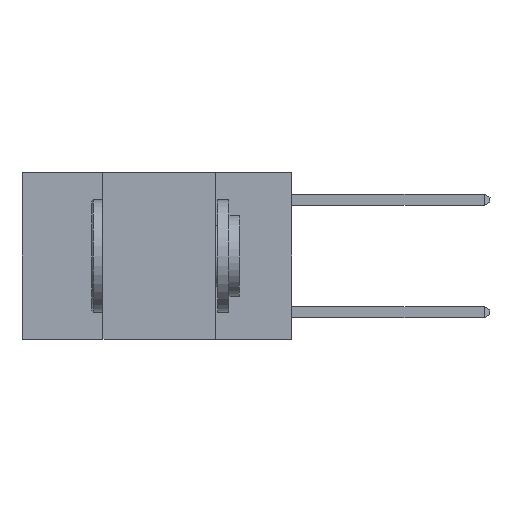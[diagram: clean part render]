
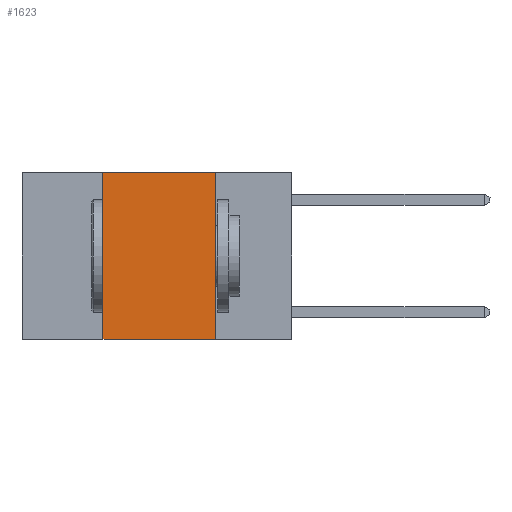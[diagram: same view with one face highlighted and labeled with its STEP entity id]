
A CAD part, left-side view. The second image highlights one B-rep face of the part: STEP entity #1623.
In plain terms, the highlighted planar face has unit normal (-1, 0, 0).
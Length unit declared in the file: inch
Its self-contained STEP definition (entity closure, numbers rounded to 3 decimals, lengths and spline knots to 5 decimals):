
#949 = CARTESIAN_POINT ( 'NONE',  ( 0., 0.17, 0. ) ) ;
#995 = CARTESIAN_POINT ( 'NONE',  ( 0., 0.6, -0.37 ) ) ;
#1240 = CARTESIAN_POINT ( 'NONE',  ( 0., 0.6, 0. ) ) ;
#1572 = DIRECTION ( 'NONE',  ( 0., 0., -1. ) ) ;
#1623 = ADVANCED_FACE ( 'NONE', ( #8697 ), #2121, .F. ) ;
#1650 = EDGE_CURVE ( 'NONE', #4309, #4981, #1725, .T. ) ;
#1725 = LINE ( 'NONE', #995, #6433 ) ;
#2109 = LINE ( 'NONE', #1240, #7111 ) ;
#2121 = PLANE ( 'NONE',  #3975 ) ;
#2131 = ORIENTED_EDGE ( 'NONE', *, *, #5411, .F. ) ;
#2407 = ORIENTED_EDGE ( 'NONE', *, *, #1650, .T. ) ;
#2868 = CARTESIAN_POINT ( 'NONE',  ( 0., 0.17, 0. ) ) ;
#3050 = VECTOR ( 'NONE', #1572, 39.37008 ) ;
#3256 = DIRECTION ( 'NONE',  ( 0., -1., 0. ) ) ;
#3333 = CARTESIAN_POINT ( 'NONE',  ( 0., 0.42, 0. ) ) ;
#3726 = ORIENTED_EDGE ( 'NONE', *, *, #3736, .F. ) ;
#3736 = EDGE_CURVE ( 'NONE', #5760, #6462, #2109, .T. ) ;
#3975 = AXIS2_PLACEMENT_3D ( 'NONE', #5078, #7504, #4783 ) ;
#4120 = CARTESIAN_POINT ( 'NONE',  ( 0., 0.17, -0.37 ) ) ;
#4208 = EDGE_LOOP ( 'NONE', ( #4667, #3726, #2131, #2407 ) ) ;
#4309 = VERTEX_POINT ( 'NONE', #5350 ) ;
#4667 = ORIENTED_EDGE ( 'NONE', *, *, #5664, .F. ) ;
#4783 = DIRECTION ( 'NONE',  ( 0., 0., -1. ) ) ;
#4833 = CARTESIAN_POINT ( 'NONE',  ( 0., 0.42, 0. ) ) ;
#4981 = VERTEX_POINT ( 'NONE', #4120 ) ;
#5078 = CARTESIAN_POINT ( 'NONE',  ( 0., 0.6, 0. ) ) ;
#5350 = CARTESIAN_POINT ( 'NONE',  ( 0., 0.42, -0.37 ) ) ;
#5354 = VECTOR ( 'NONE', #5598, 39.37008 ) ;
#5411 = EDGE_CURVE ( 'NONE', #4309, #5760, #9169, .T. ) ;
#5598 = DIRECTION ( 'NONE',  ( 0., 0., 1. ) ) ;
#5664 = EDGE_CURVE ( 'NONE', #6462, #4981, #8167, .T. ) ;
#5760 = VERTEX_POINT ( 'NONE', #3333 ) ;
#6433 = VECTOR ( 'NONE', #3256, 39.37008 ) ;
#6462 = VERTEX_POINT ( 'NONE', #2868 ) ;
#7111 = VECTOR ( 'NONE', #9450, 39.37008 ) ;
#7504 = DIRECTION ( 'NONE',  ( 1., 0., 0. ) ) ;
#8167 = LINE ( 'NONE', #949, #3050 ) ;
#8697 = FACE_OUTER_BOUND ( 'NONE', #4208, .T. ) ;
#9169 = LINE ( 'NONE', #4833, #5354 ) ;
#9450 = DIRECTION ( 'NONE',  ( 0., -1., 0. ) ) ;
